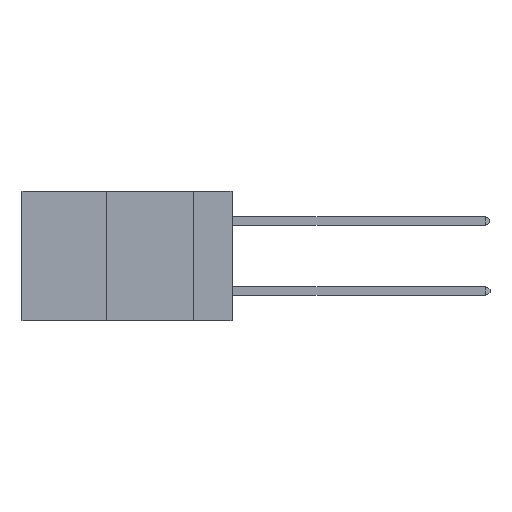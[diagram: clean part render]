
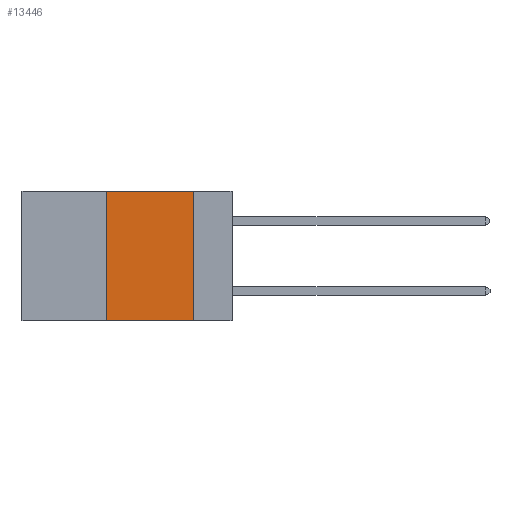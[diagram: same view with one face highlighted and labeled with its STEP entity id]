
A CAD part, left-side view. The second image highlights one B-rep face of the part: STEP entity #13446.
In plain terms, the highlighted planar face has unit normal (-1, 0, 0).
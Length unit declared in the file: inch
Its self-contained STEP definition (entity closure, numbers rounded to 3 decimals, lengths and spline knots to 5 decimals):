
#122 = DIRECTION ( 'NONE',  ( 0., 0., 1. ) ) ;
#420 = CARTESIAN_POINT ( 'NONE',  ( 0., 0.6, 0. ) ) ;
#1742 = ORIENTED_EDGE ( 'NONE', *, *, #5471, .F. ) ;
#2255 = ORIENTED_EDGE ( 'NONE', *, *, #15616, .F. ) ;
#2728 = CARTESIAN_POINT ( 'NONE',  ( 0., 0.36, -0.37 ) ) ;
#3509 = PLANE ( 'NONE',  #5773 ) ;
#4696 = VERTEX_POINT ( 'NONE', #19408 ) ;
#5471 = EDGE_CURVE ( 'NONE', #20255, #22440, #23293, .T. ) ;
#5773 = AXIS2_PLACEMENT_3D ( 'NONE', #10746, #18917, #6392 ) ;
#6392 = DIRECTION ( 'NONE',  ( 0., 0., -1. ) ) ;
#6501 = EDGE_LOOP ( 'NONE', ( #1742, #12666, #2255, #13474 ) ) ;
#7428 = VECTOR ( 'NONE', #13361, 39.37008 ) ;
#8978 = LINE ( 'NONE', #17482, #7428 ) ;
#9686 = CARTESIAN_POINT ( 'NONE',  ( 0., 0.36, 0. ) ) ;
#9995 = CARTESIAN_POINT ( 'NONE',  ( 0., 0.11, -0.37 ) ) ;
#10746 = CARTESIAN_POINT ( 'NONE',  ( 0., 0.6, 0. ) ) ;
#11523 = FACE_OUTER_BOUND ( 'NONE', #6501, .T. ) ;
#12041 = VECTOR ( 'NONE', #122, 39.37008 ) ;
#12666 = ORIENTED_EDGE ( 'NONE', *, *, #19093, .F. ) ;
#13361 = DIRECTION ( 'NONE',  ( 0., -1., 0. ) ) ;
#13364 = LINE ( 'NONE', #420, #19776 ) ;
#13446 = ADVANCED_FACE ( 'NONE', ( #11523 ), #3509, .F. ) ;
#13474 = ORIENTED_EDGE ( 'NONE', *, *, #22862, .T. ) ;
#15457 = CARTESIAN_POINT ( 'NONE',  ( 0., 0.11, 0. ) ) ;
#15616 = EDGE_CURVE ( 'NONE', #21327, #4696, #22415, .T. ) ;
#17247 = DIRECTION ( 'NONE',  ( 0., 0., -1. ) ) ;
#17482 = CARTESIAN_POINT ( 'NONE',  ( 0., 0.6, -0.37 ) ) ;
#17679 = CARTESIAN_POINT ( 'NONE',  ( 0., 0.11, 0. ) ) ;
#17904 = DIRECTION ( 'NONE',  ( 0., -1., 0. ) ) ;
#18087 = VECTOR ( 'NONE', #17247, 39.37008 ) ;
#18917 = DIRECTION ( 'NONE',  ( 1., 0., 0. ) ) ;
#19093 = EDGE_CURVE ( 'NONE', #4696, #20255, #13364, .T. ) ;
#19408 = CARTESIAN_POINT ( 'NONE',  ( 0., 0.36, 0. ) ) ;
#19776 = VECTOR ( 'NONE', #17904, 39.37008 ) ;
#20255 = VERTEX_POINT ( 'NONE', #17679 ) ;
#21327 = VERTEX_POINT ( 'NONE', #2728 ) ;
#22415 = LINE ( 'NONE', #9686, #12041 ) ;
#22440 = VERTEX_POINT ( 'NONE', #9995 ) ;
#22862 = EDGE_CURVE ( 'NONE', #21327, #22440, #8978, .T. ) ;
#23293 = LINE ( 'NONE', #15457, #18087 ) ;
